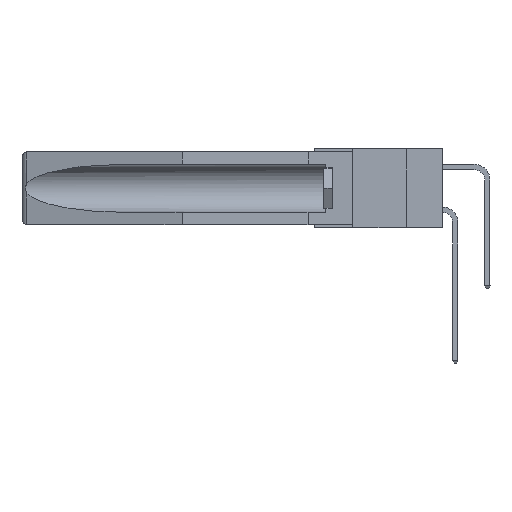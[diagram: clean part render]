
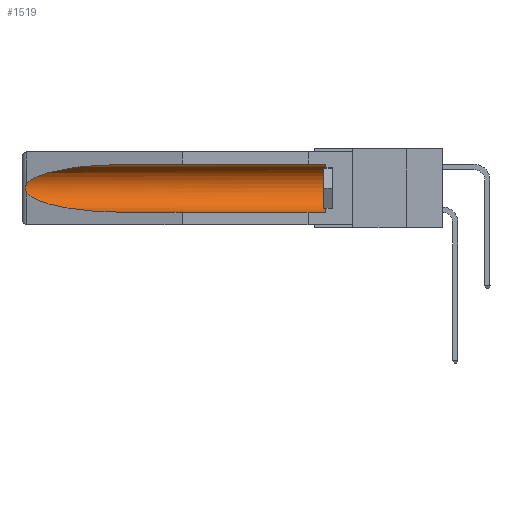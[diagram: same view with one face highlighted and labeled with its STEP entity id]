
A CAD part, left-side view. The second image highlights one B-rep face of the part: STEP entity #1519.
In plain terms, the highlighted cylindrical face has radius 2.857 mm (diameter 5.715 mm), a partial arc.
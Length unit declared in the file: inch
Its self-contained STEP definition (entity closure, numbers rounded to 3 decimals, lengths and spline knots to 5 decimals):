
#592 = CARTESIAN_POINT ( 'NONE',  ( 0.21114, 1.30732, -0.059 ) ) ;
#1519 = ADVANCED_FACE ( 'NONE', ( #6965 ), #2479, .F. ) ;
#1943 = AXIS2_PLACEMENT_3D ( 'NONE', #13896, #17381, #12010 ) ;
#1947 =( BOUNDED_CURVE ( )  B_SPLINE_CURVE ( 3, ( #7182, #20845, #2149, #3862 ),
 .UNSPECIFIED., .F., .F. ) 
 B_SPLINE_CURVE_WITH_KNOTS ( ( 4, 4 ),
 ( 0.1948, 1.5708 ),
 .UNSPECIFIED. ) 
 CURVE ( )  GEOMETRIC_REPRESENTATION_ITEM ( )  RATIONAL_B_SPLINE_CURVE ( ( 1., 0.848, 0.848, 1. ) ) 
 REPRESENTATION_ITEM ( '' )  );
#2129 = CARTESIAN_POINT ( 'NONE',  ( 0.155, 1.07973, -0.059 ) ) ;
#2149 = CARTESIAN_POINT ( 'NONE',  ( 0.21114, 1.30732, -0.284 ) ) ;
#2479 = CYLINDRICAL_SURFACE ( 'NONE', #21276, 0.1125 ) ;
#2789 = LINE ( 'NONE', #10898, #11281 ) ;
#3011 = CARTESIAN_POINT ( 'NONE',  ( 0.155, 0.126, -0.059 ) ) ;
#3581 = CARTESIAN_POINT ( 'NONE',  ( 0.155, 0.126, -0.284 ) ) ;
#3862 = CARTESIAN_POINT ( 'NONE',  ( 0.155, 1.07973, -0.284 ) ) ;
#3920 =( BOUNDED_CURVE ( )  B_SPLINE_CURVE ( 3, ( #13936, #592, #7206, #3966 ),
 .UNSPECIFIED., .F., .F. ) 
 B_SPLINE_CURVE_WITH_KNOTS ( ( 4, 4 ),
 ( 4.71239, 6.08839 ),
 .UNSPECIFIED. ) 
 CURVE ( )  GEOMETRIC_REPRESENTATION_ITEM ( )  RATIONAL_B_SPLINE_CURVE ( ( 1., 0.848, 0.848, 1. ) ) 
 REPRESENTATION_ITEM ( '' )  );
#3966 = CARTESIAN_POINT ( 'NONE',  ( 0.26537, 1.52718, -0.14972 ) ) ;
#4393 = VERTEX_POINT ( 'NONE', #12231 ) ;
#4447 = CARTESIAN_POINT ( 'NONE',  ( 0.2675, 1.53308, -0.16763 ) ) ;
#4995 = EDGE_CURVE ( 'NONE', #4393, #5773, #1947, .T. ) ;
#5773 = VERTEX_POINT ( 'NONE', #14384 ) ;
#6139 = CARTESIAN_POINT ( 'NONE',  ( 0.26537, 1.52718, -0.19328 ) ) ;
#6965 = FACE_OUTER_BOUND ( 'NONE', #21681, .T. ) ;
#7182 = CARTESIAN_POINT ( 'NONE',  ( 0.26537, 1.52718, -0.19328 ) ) ;
#7206 = CARTESIAN_POINT ( 'NONE',  ( 0.25451, 1.48313, -0.09465 ) ) ;
#7828 = LINE ( 'NONE', #20971, #9173 ) ;
#8441 = ORIENTED_EDGE ( 'NONE', *, *, #14518, .F. ) ;
#8473 = CARTESIAN_POINT ( 'NONE',  ( 0.155, -0.30754, -0.1715 ) ) ;
#9086 = ORIENTED_EDGE ( 'NONE', *, *, #4995, .T. ) ;
#9173 = VECTOR ( 'NONE', #12612, 39.37008 ) ;
#9515 = EDGE_CURVE ( 'NONE', #11346, #17119, #19738, .T. ) ;
#9567 = DIRECTION ( 'NONE',  ( 0., 1., 0. ) ) ;
#9571 = CARTESIAN_POINT ( 'NONE',  ( 0.26655, 1.53094, -0.18657 ) ) ;
#10115 = DIRECTION ( 'NONE',  ( 0., 0., 1. ) ) ;
#10159 = VERTEX_POINT ( 'NONE', #15722 ) ;
#10194 = ORIENTED_EDGE ( 'NONE', *, *, #21220, .T. ) ;
#10898 = CARTESIAN_POINT ( 'NONE',  ( 0.155, -0.30754, -0.059 ) ) ;
#11114 = CARTESIAN_POINT ( 'NONE',  ( 0.2675, 1.53308, -0.17534 ) ) ;
#11198 = CARTESIAN_POINT ( 'NONE',  ( 0.26537, 1.52718, -0.14972 ) ) ;
#11281 = VECTOR ( 'NONE', #9567, 39.37008 ) ;
#11346 = VERTEX_POINT ( 'NONE', #3581 ) ;
#12010 = DIRECTION ( 'NONE',  ( 0., 0., 1. ) ) ;
#12231 = CARTESIAN_POINT ( 'NONE',  ( 0.26537, 1.52718, -0.19328 ) ) ;
#12612 = DIRECTION ( 'NONE',  ( 0., 1., 0. ) ) ;
#13896 = CARTESIAN_POINT ( 'NONE',  ( 0.155, 0.126, -0.1715 ) ) ;
#13936 = CARTESIAN_POINT ( 'NONE',  ( 0.155, 1.07973, -0.059 ) ) ;
#14384 = CARTESIAN_POINT ( 'NONE',  ( 0.155, 1.07973, -0.284 ) ) ;
#14518 = EDGE_CURVE ( 'NONE', #11346, #5773, #7828, .T. ) ;
#14632 = CARTESIAN_POINT ( 'NONE',  ( 0.26654, 1.53092, -0.15636 ) ) ;
#14965 = DIRECTION ( 'NONE',  ( 0., 1., 0. ) ) ;
#15722 = CARTESIAN_POINT ( 'NONE',  ( 0.26537, 1.52718, -0.14972 ) ) ;
#16323 = CARTESIAN_POINT ( 'NONE',  ( 0.26597, 1.5296, -0.19026 ) ) ;
#16884 = ORIENTED_EDGE ( 'NONE', *, *, #17696, .T. ) ;
#16945 = VERTEX_POINT ( 'NONE', #2129 ) ;
#17076 = B_SPLINE_CURVE_WITH_KNOTS ( 'NONE', 3,
 ( #11198, #17761, #14632, #17910, #4447, #11114, #19490, #9571, #16323, #6139 ),
 .UNSPECIFIED., .F., .F.,
 ( 4, 2, 2, 2, 4 ),
 ( 0., 0.00029, 0.00058, 0.00087, 0.00117 ),
 .UNSPECIFIED. ) ;
#17119 = VERTEX_POINT ( 'NONE', #3011 ) ;
#17381 = DIRECTION ( 'NONE',  ( 0., -1., 0. ) ) ;
#17696 = EDGE_CURVE ( 'NONE', #10159, #4393, #17076, .T. ) ;
#17761 = CARTESIAN_POINT ( 'NONE',  ( 0.26597, 1.52961, -0.15275 ) ) ;
#17910 = CARTESIAN_POINT ( 'NONE',  ( 0.2673, 1.5327, -0.16383 ) ) ;
#19180 = ORIENTED_EDGE ( 'NONE', *, *, #20439, .T. ) ;
#19490 = CARTESIAN_POINT ( 'NONE',  ( 0.2673, 1.53269, -0.17917 ) ) ;
#19738 = CIRCLE ( 'NONE', #1943, 0.1125 ) ;
#19882 = ORIENTED_EDGE ( 'NONE', *, *, #9515, .T. ) ;
#20439 = EDGE_CURVE ( 'NONE', #17119, #16945, #2789, .T. ) ;
#20845 = CARTESIAN_POINT ( 'NONE',  ( 0.25451, 1.48313, -0.24835 ) ) ;
#20971 = CARTESIAN_POINT ( 'NONE',  ( 0.155, -0.30754, -0.284 ) ) ;
#21220 = EDGE_CURVE ( 'NONE', #16945, #10159, #3920, .T. ) ;
#21276 = AXIS2_PLACEMENT_3D ( 'NONE', #8473, #14965, #10115 ) ;
#21681 = EDGE_LOOP ( 'NONE', ( #10194, #16884, #9086, #8441, #19882, #19180 ) ) ;
